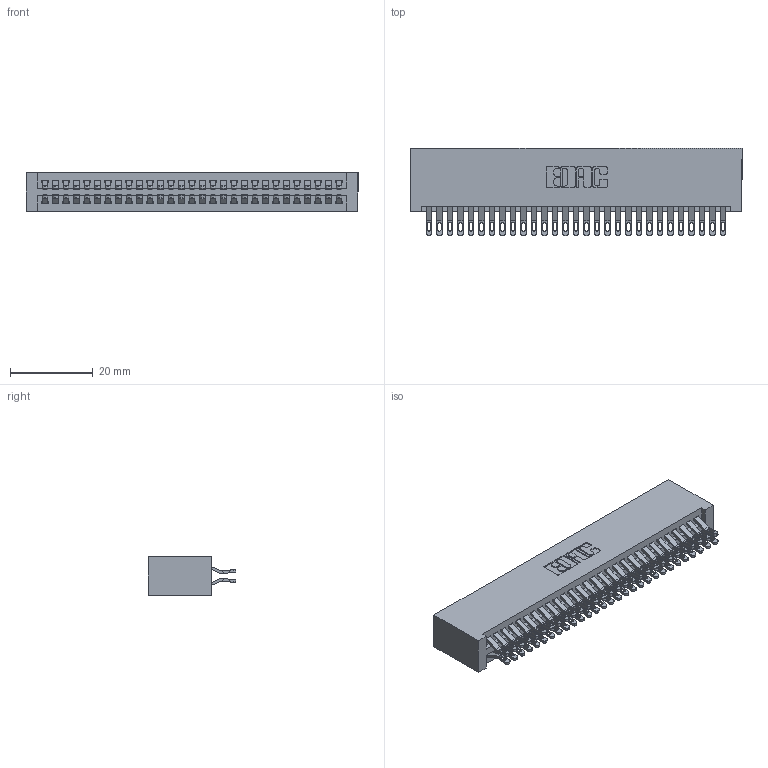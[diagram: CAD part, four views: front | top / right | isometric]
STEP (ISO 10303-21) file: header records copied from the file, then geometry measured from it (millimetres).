
FILE_DESCRIPTION (( 'STEP AP203' ), '1' );
FILE_NAME ('395-058-555-201.STEP', '2018-11-23T04:28:56', ( '' ), ( '' ), 'SwSTEP 2.0', 'SolidWorks 2016', '' );
FILE_SCHEMA (( 'CONFIG_CONTROL_DESIGN' ));
Length unit declared in the file: inch
Products named in the file (3): 345-292-001_555 Tail; 345 Part_No Mounting Lugs; 395-058-555-201
Assembly tree (59 placements, depth 2):
  395-058-555-201
    345 Part_No Mounting Lugs
    345-292-001_555 Tail  x58
Bounding box: 80.26 x 21.13 x 9.4 mm (x, y, z)
Volume: 8460.4 mm3; surface area: 13142.5 mm2
Topology: 59 solids, 59 shells, 3366 faces, 10583 edges, 7054 vertices
Faces by surface type: plane 1874, cylinder 1492
Entity records: 24553 total; most frequent: CARTESIAN_POINT 4162, ORIENTED_EDGE 4066, DIRECTION 3649, EDGE_CURVE 2033, VECTOR 1773, LINE 1773, VERTEX_POINT 1354, AXIS2_PLACEMENT_3D 938
